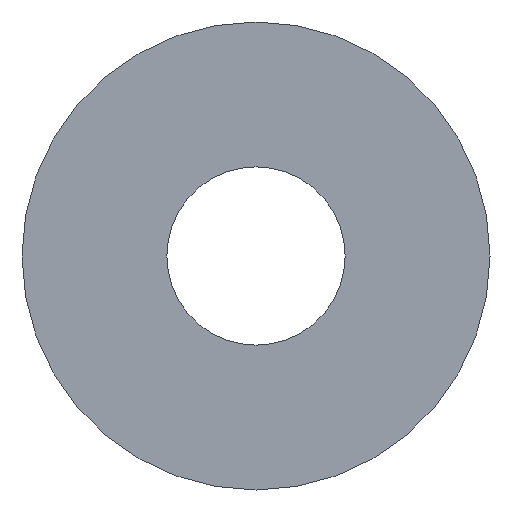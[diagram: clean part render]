
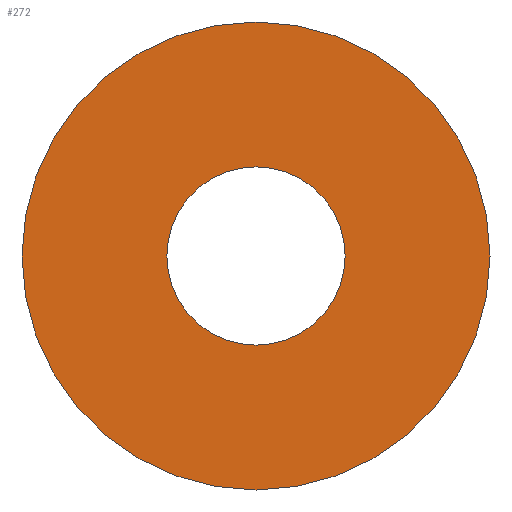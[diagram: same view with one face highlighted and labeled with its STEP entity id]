
A CAD part, front view. The second image highlights one B-rep face of the part: STEP entity #272.
In plain terms, the highlighted planar face has unit normal (0, -1, 0).
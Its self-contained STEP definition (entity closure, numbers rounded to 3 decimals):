
#25 = ORIENTED_EDGE ( 'NONE', *, *, #284, .F. ) ;
#56 = DIRECTION ( 'NONE',  ( 0., 0., -1. ) ) ;
#57 = DIRECTION ( 'NONE',  ( 0., -1., 0. ) ) ;
#61 = CARTESIAN_POINT ( 'NONE',  ( 0., -1.555, 0. ) ) ;
#62 = DIRECTION ( 'NONE',  ( 0., 0., -1. ) ) ;
#63 = DIRECTION ( 'NONE',  ( 0., -1., 0. ) ) ;
#64 = CARTESIAN_POINT ( 'NONE',  ( 0., -1.555, 0. ) ) ;
#74 = DIRECTION ( 'NONE',  ( 0., 0., -1. ) ) ;
#75 = DIRECTION ( 'NONE',  ( 0., -1., 0. ) ) ;
#76 = CARTESIAN_POINT ( 'NONE',  ( 0., -1.555, 0. ) ) ;
#86 = DIRECTION ( 'NONE',  ( 0., 0., -1. ) ) ;
#87 = DIRECTION ( 'NONE',  ( 0., -1., 0. ) ) ;
#88 = CARTESIAN_POINT ( 'NONE',  ( 0., -1.555, 0. ) ) ;
#111 = DIRECTION ( 'NONE',  ( 0., 0., -1. ) ) ;
#112 = DIRECTION ( 'NONE',  ( 0., -1., 0. ) ) ;
#113 = CARTESIAN_POINT ( 'NONE',  ( 2., -1.555, 0. ) ) ;
#114 = PLANE ( 'NONE',  #199 ) ;
#131 = CARTESIAN_POINT ( 'NONE',  ( 0., -1.555, -2. ) ) ;
#132 = CARTESIAN_POINT ( 'NONE',  ( 0., -1.555, 2. ) ) ;
#135 = CARTESIAN_POINT ( 'NONE',  ( 0., -1.555, -5.25 ) ) ;
#136 = CARTESIAN_POINT ( 'NONE',  ( 0., -1.555, 5.25 ) ) ;
#159 = VERTEX_POINT ( 'NONE', #136 ) ;
#161 = VERTEX_POINT ( 'NONE', #135 ) ;
#165 = ORIENTED_EDGE ( 'NONE', *, *, #290, .T. ) ;
#166 = VERTEX_POINT ( 'NONE', #132 ) ;
#167 = VERTEX_POINT ( 'NONE', #131 ) ;
#172 = EDGE_LOOP ( 'NONE', ( #182, #25 ) ) ;
#178 = EDGE_LOOP ( 'NONE', ( #196, #165 ) ) ;
#182 = ORIENTED_EDGE ( 'NONE', *, *, #288, .F. ) ;
#196 = ORIENTED_EDGE ( 'NONE', *, *, #280, .T. ) ;
#199 = AXIS2_PLACEMENT_3D ( 'NONE', #113, #112, #111 ) ;
#201 = FACE_BOUND ( 'NONE', #172, .T. ) ;
#221 = FACE_OUTER_BOUND ( 'NONE', #178, .T. ) ;
#229 = AXIS2_PLACEMENT_3D ( 'NONE', #76, #75, #74 ) ;
#233 = AXIS2_PLACEMENT_3D ( 'NONE', #61, #57, #56 ) ;
#240 = AXIS2_PLACEMENT_3D ( 'NONE', #88, #87, #86 ) ;
#248 = AXIS2_PLACEMENT_3D ( 'NONE', #64, #63, #62 ) ;
#257 = CIRCLE ( 'NONE', #233, 5.25 ) ;
#258 = CIRCLE ( 'NONE', #248, 2. ) ;
#263 = CIRCLE ( 'NONE', #240, 5.25 ) ;
#264 = CIRCLE ( 'NONE', #229, 2. ) ;
#272 = ADVANCED_FACE ( 'NONE', ( #221, #201 ), #114, .T. ) ;
#280 = EDGE_CURVE ( 'NONE', #161, #159, #263, .T. ) ;
#284 = EDGE_CURVE ( 'NONE', #166, #167, #264, .T. ) ;
#288 = EDGE_CURVE ( 'NONE', #167, #166, #258, .T. ) ;
#290 = EDGE_CURVE ( 'NONE', #159, #161, #257, .T. ) ;
